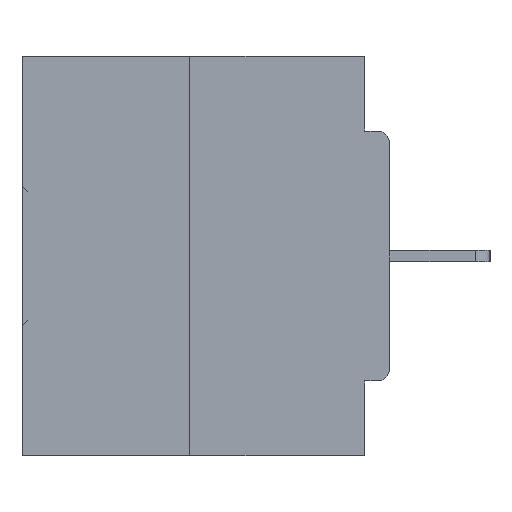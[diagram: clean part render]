
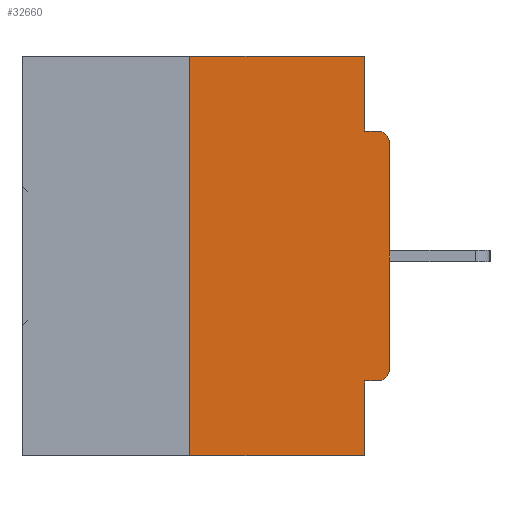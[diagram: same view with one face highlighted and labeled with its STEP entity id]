
A CAD part, left-side view. The second image highlights one B-rep face of the part: STEP entity #32660.
In plain terms, the highlighted planar face has unit normal (-1, 0, 0).
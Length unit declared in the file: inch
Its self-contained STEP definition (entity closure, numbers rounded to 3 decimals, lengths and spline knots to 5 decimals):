
#490 = CARTESIAN_POINT ( 'NONE',  ( 0., 0.25, 0. ) ) ;
#886 = CARTESIAN_POINT ( 'NONE',  ( 0., 0., -0.4065 ) ) ;
#1199 = AXIS2_PLACEMENT_3D ( 'NONE', #25746, #7310, #28764 ) ;
#1619 = CARTESIAN_POINT ( 'NONE',  ( 0., 0.46, 0. ) ) ;
#3108 = VERTEX_POINT ( 'NONE', #9493 ) ;
#3446 = DIRECTION ( 'NONE',  ( 0., 0., -1. ) ) ;
#3745 = ORIENTED_EDGE ( 'NONE', *, *, #32844, .F. ) ;
#4043 = DIRECTION ( 'NONE',  ( 0., 1., 0. ) ) ;
#4054 = ORIENTED_EDGE ( 'NONE', *, *, #6778, .F. ) ;
#4107 = ORIENTED_EDGE ( 'NONE', *, *, #34847, .T. ) ;
#4184 = ORIENTED_EDGE ( 'NONE', *, *, #8335, .F. ) ;
#4676 = ORIENTED_EDGE ( 'NONE', *, *, #7800, .F. ) ;
#4716 = ORIENTED_EDGE ( 'NONE', *, *, #11737, .T. ) ;
#4773 = VERTEX_POINT ( 'NONE', #16537 ) ;
#5088 = CARTESIAN_POINT ( 'NONE',  ( 0., 0.46, -0.5 ) ) ;
#5230 = ORIENTED_EDGE ( 'NONE', *, *, #37828, .T. ) ;
#5252 = LINE ( 'NONE', #38383, #20842 ) ;
#5260 = ORIENTED_EDGE ( 'NONE', *, *, #17688, .T. ) ;
#5637 = ORIENTED_EDGE ( 'NONE', *, *, #28606, .F. ) ;
#5702 = CARTESIAN_POINT ( 'NONE',  ( 0., 0.031, 0. ) ) ;
#5744 = ORIENTED_EDGE ( 'NONE', *, *, #34342, .F. ) ;
#6494 = VECTOR ( 'NONE', #3446, 39.37008 ) ;
#6778 = EDGE_CURVE ( 'NONE', #3108, #24793, #16445, .T. ) ;
#7310 = DIRECTION ( 'NONE',  ( -1., 0., 0. ) ) ;
#7497 = FACE_OUTER_BOUND ( 'NONE', #21530, .T. ) ;
#7800 = EDGE_CURVE ( 'NONE', #14026, #8451, #26768, .T. ) ;
#7885 = LINE ( 'NONE', #14892, #38249 ) ;
#8232 = DIRECTION ( 'NONE',  ( 0., -1., 0. ) ) ;
#8335 = EDGE_CURVE ( 'NONE', #8451, #22713, #30989, .T. ) ;
#8451 = VERTEX_POINT ( 'NONE', #22890 ) ;
#9099 = CARTESIAN_POINT ( 'NONE',  ( 0., 0.015, -0.1085 ) ) ;
#9493 = CARTESIAN_POINT ( 'NONE',  ( 0., 0.25, -0.5 ) ) ;
#10166 = CARTESIAN_POINT ( 'NONE',  ( 0., 0., -0.3915 ) ) ;
#11295 = VECTOR ( 'NONE', #8232, 39.37008 ) ;
#11737 = EDGE_CURVE ( 'NONE', #14026, #31478, #21815, .T. ) ;
#12295 = DIRECTION ( 'NONE',  ( 0., 0., -1. ) ) ;
#13371 = CARTESIAN_POINT ( 'NONE',  ( 0., 0.46, 0. ) ) ;
#14026 = VERTEX_POINT ( 'NONE', #33287 ) ;
#14398 = VECTOR ( 'NONE', #30362, 39.37008 ) ;
#14540 = CARTESIAN_POINT ( 'NONE',  ( 0., 0.031, -0.5 ) ) ;
#14892 = CARTESIAN_POINT ( 'NONE',  ( 0., 0.031, 0. ) ) ;
#16297 = LINE ( 'NONE', #1619, #39227 ) ;
#16445 = LINE ( 'NONE', #26412, #30637 ) ;
#16481 = PLANE ( 'NONE',  #35172 ) ;
#16537 = CARTESIAN_POINT ( 'NONE',  ( 0., 0.031, -0.0935 ) ) ;
#17688 = EDGE_CURVE ( 'NONE', #37197, #30024, #19602, .T. ) ;
#17807 = VECTOR ( 'NONE', #4043, 39.37008 ) ;
#18142 = CARTESIAN_POINT ( 'NONE',  ( 0., 0., -0.1085 ) ) ;
#19535 = DIRECTION ( 'NONE',  ( 0., 0., -1. ) ) ;
#19602 = CIRCLE ( 'NONE', #36471, 0.015 ) ;
#20509 = DIRECTION ( 'NONE',  ( 0., 0., 1. ) ) ;
#20842 = VECTOR ( 'NONE', #29506, 39.37008 ) ;
#21349 = CARTESIAN_POINT ( 'NONE',  ( 0., 0.015, -0.0935 ) ) ;
#21530 = EDGE_LOOP ( 'NONE', ( #3745, #4054, #4107, #4184, #4676, #4716, #5230, #5260, #5637, #5744 ) ) ;
#21815 = CIRCLE ( 'NONE', #1199, 0.015 ) ;
#22713 = VERTEX_POINT ( 'NONE', #14540 ) ;
#22890 = CARTESIAN_POINT ( 'NONE',  ( 0., 0.031, -0.4065 ) ) ;
#24793 = VERTEX_POINT ( 'NONE', #490 ) ;
#25477 = DIRECTION ( 'NONE',  ( 1., 0., 0. ) ) ;
#25746 = CARTESIAN_POINT ( 'NONE',  ( 0., 0.015, -0.3915 ) ) ;
#26412 = CARTESIAN_POINT ( 'NONE',  ( 0., 0.25, 0. ) ) ;
#26768 = LINE ( 'NONE', #886, #17807 ) ;
#27303 = CARTESIAN_POINT ( 'NONE',  ( 0., 0., 0. ) ) ;
#27996 = CARTESIAN_POINT ( 'NONE',  ( 0., 0.031, -0.5 ) ) ;
#28606 = EDGE_CURVE ( 'NONE', #4773, #30024, #5252, .T. ) ;
#28764 = DIRECTION ( 'NONE',  ( 0., 0., -1. ) ) ;
#29506 = DIRECTION ( 'NONE',  ( 0., -1., 0. ) ) ;
#30024 = VERTEX_POINT ( 'NONE', #21349 ) ;
#30362 = DIRECTION ( 'NONE',  ( 0., 0., 1. ) ) ;
#30530 = DIRECTION ( 'NONE',  ( -1., 0., 0. ) ) ;
#30637 = VECTOR ( 'NONE', #20509, 39.37008 ) ;
#30989 = LINE ( 'NONE', #27996, #6494 ) ;
#31478 = VERTEX_POINT ( 'NONE', #10166 ) ;
#32660 = ADVANCED_FACE ( 'NONE', ( #7497 ), #16481, .F. ) ;
#32844 = EDGE_CURVE ( 'NONE', #24793, #37212, #16297, .T. ) ;
#33287 = CARTESIAN_POINT ( 'NONE',  ( 0., 0.015, -0.4065 ) ) ;
#34342 = EDGE_CURVE ( 'NONE', #37212, #4773, #7885, .T. ) ;
#34847 = EDGE_CURVE ( 'NONE', #3108, #22713, #35428, .T. ) ;
#35172 = AXIS2_PLACEMENT_3D ( 'NONE', #13371, #25477, #19535 ) ;
#35428 = LINE ( 'NONE', #5088, #11295 ) ;
#36471 = AXIS2_PLACEMENT_3D ( 'NONE', #9099, #30530, #12295 ) ;
#37197 = VERTEX_POINT ( 'NONE', #18142 ) ;
#37212 = VERTEX_POINT ( 'NONE', #5702 ) ;
#37828 = EDGE_CURVE ( 'NONE', #31478, #37197, #38346, .T. ) ;
#38249 = VECTOR ( 'NONE', #38995, 39.37008 ) ;
#38331 = DIRECTION ( 'NONE',  ( 0., -1., 0. ) ) ;
#38346 = LINE ( 'NONE', #27303, #14398 ) ;
#38383 = CARTESIAN_POINT ( 'NONE',  ( 0., 0., -0.0935 ) ) ;
#38995 = DIRECTION ( 'NONE',  ( 0., 0., -1. ) ) ;
#39227 = VECTOR ( 'NONE', #38331, 39.37008 ) ;
